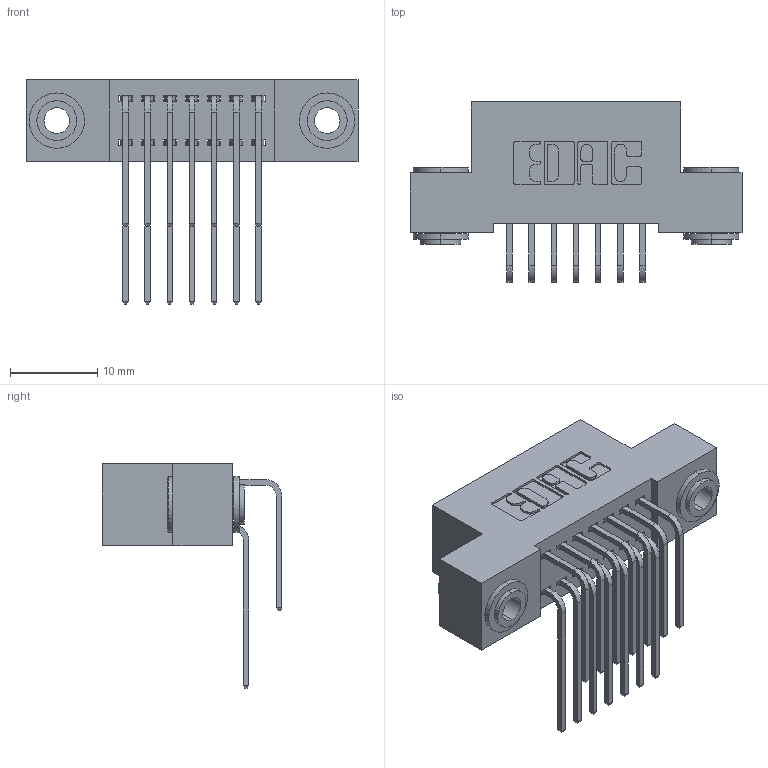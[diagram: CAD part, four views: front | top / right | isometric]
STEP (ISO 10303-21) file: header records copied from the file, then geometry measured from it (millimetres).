
FILE_DESCRIPTION (( 'STEP AP203' ), '1' );
FILE_NAME ('342-014-559-203.STEP', '2018-08-10T18:39:13', ( '' ), ( '' ), 'SwSTEP 2.0', 'SolidWorks 2016', '' );
FILE_SCHEMA (( 'CONFIG_CONTROL_DESIGN' ));
Length unit declared in the file: inch
Products named in the file (5): 342-014-559-203; 342 Part_.156 TH; 345-292-001_558 559 Tail - 1; 345-292-001_559 Tail - 2; 342-250-002_345-250-002-102
Assembly tree (17 placements, depth 2):
  342-014-559-203
    342 Part_.156 TH
    345-292-001_558 559 Tail - 1  x7
    345-292-001_559 Tail - 2  x7
    342-250-002_345-250-002-102  x2
Bounding box: 38.1 x 20.64 x 25.78 mm (x, y, z)
Volume: 3361.2 mm3; surface area: 5188.2 mm2
Topology: 17 solids, 17 shells, 904 faces, 2629 edges, 1730 vertices
Faces by surface type: plane 608, cylinder 288, cone 8
Entity records: 11332 total; most frequent: CARTESIAN_POINT 1944, ORIENTED_EDGE 1822, DIRECTION 1737, EDGE_CURVE 911, LINE 719, VECTOR 719, VERTEX_POINT 602, AXIS2_PLACEMENT_3D 509
